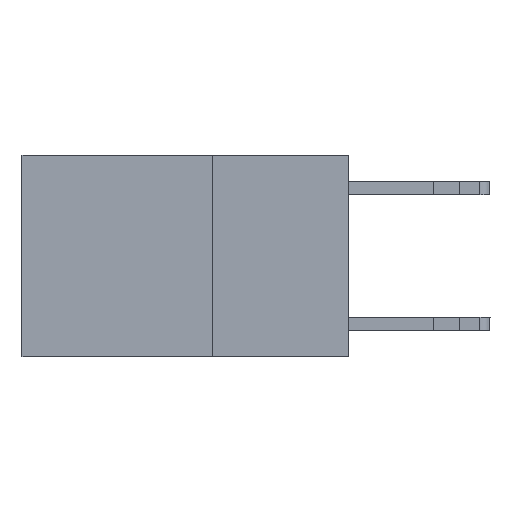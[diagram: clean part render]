
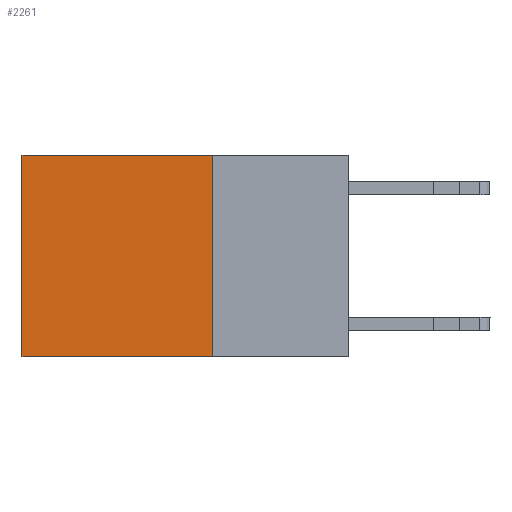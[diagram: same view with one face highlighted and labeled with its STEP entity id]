
A CAD part, left-side view. The second image highlights one B-rep face of the part: STEP entity #2261.
In plain terms, the highlighted planar face has unit normal (-1, 0, 0).
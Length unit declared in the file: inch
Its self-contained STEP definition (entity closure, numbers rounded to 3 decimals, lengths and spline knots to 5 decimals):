
#1260 = CARTESIAN_POINT ( 'NONE',  ( 0.2625, 0.25, -0.37 ) ) ;
#1517 = ORIENTED_EDGE ( 'NONE', *, *, #8712, .T. ) ;
#1539 = ORIENTED_EDGE ( 'NONE', *, *, #15806, .T. ) ;
#1638 = CARTESIAN_POINT ( 'NONE',  ( 0.2625, 0.25, 0. ) ) ;
#1771 = DIRECTION ( 'NONE',  ( 0., 0., -1. ) ) ;
#2261 = ADVANCED_FACE ( 'NONE', ( #9643 ), #4360, .F. ) ;
#2660 = LINE ( 'NONE', #3826, #6654 ) ;
#2894 = CARTESIAN_POINT ( 'NONE',  ( 0.2625, 0.25, -0.37 ) ) ;
#2945 = AXIS2_PLACEMENT_3D ( 'NONE', #18060, #16611, #9456 ) ;
#3750 = DIRECTION ( 'NONE',  ( 0., 0., -1. ) ) ;
#3826 = CARTESIAN_POINT ( 'NONE',  ( 0.2625, 0.6, 0. ) ) ;
#4329 = CARTESIAN_POINT ( 'NONE',  ( 0.2625, 0.6, -0.37 ) ) ;
#4360 = PLANE ( 'NONE',  #2945 ) ;
#4432 = DIRECTION ( 'NONE',  ( 0., 1., 0. ) ) ;
#4607 = VECTOR ( 'NONE', #1771, 39.37008 ) ;
#5932 = VERTEX_POINT ( 'NONE', #1638 ) ;
#6389 = DIRECTION ( 'NONE',  ( 0., 1., 0. ) ) ;
#6654 = VECTOR ( 'NONE', #3750, 39.37008 ) ;
#7955 = LINE ( 'NONE', #15156, #4607 ) ;
#8467 = ORIENTED_EDGE ( 'NONE', *, *, #17549, .F. ) ;
#8712 = EDGE_CURVE ( 'NONE', #5932, #10781, #14926, .T. ) ;
#9456 = DIRECTION ( 'NONE',  ( 0., 0., -1. ) ) ;
#9643 = FACE_OUTER_BOUND ( 'NONE', #15006, .T. ) ;
#10781 = VERTEX_POINT ( 'NONE', #17193 ) ;
#11083 = ORIENTED_EDGE ( 'NONE', *, *, #17787, .F. ) ;
#14926 = LINE ( 'NONE', #15760, #17410 ) ;
#14999 = VECTOR ( 'NONE', #4432, 39.37008 ) ;
#15006 = EDGE_LOOP ( 'NONE', ( #1539, #8467, #11083, #1517 ) ) ;
#15156 = CARTESIAN_POINT ( 'NONE',  ( 0.2625, 0.25, 0. ) ) ;
#15760 = CARTESIAN_POINT ( 'NONE',  ( 0.2625, 0.25, 0. ) ) ;
#15806 = EDGE_CURVE ( 'NONE', #10781, #17546, #2660, .T. ) ;
#16520 = VERTEX_POINT ( 'NONE', #2894 ) ;
#16611 = DIRECTION ( 'NONE',  ( 1., 0., 0. ) ) ;
#16929 = LINE ( 'NONE', #1260, #14999 ) ;
#17193 = CARTESIAN_POINT ( 'NONE',  ( 0.2625, 0.6, 0. ) ) ;
#17410 = VECTOR ( 'NONE', #6389, 39.37008 ) ;
#17546 = VERTEX_POINT ( 'NONE', #4329 ) ;
#17549 = EDGE_CURVE ( 'NONE', #16520, #17546, #16929, .T. ) ;
#17787 = EDGE_CURVE ( 'NONE', #5932, #16520, #7955, .T. ) ;
#18060 = CARTESIAN_POINT ( 'NONE',  ( 0.2625, 0.25, 0. ) ) ;
